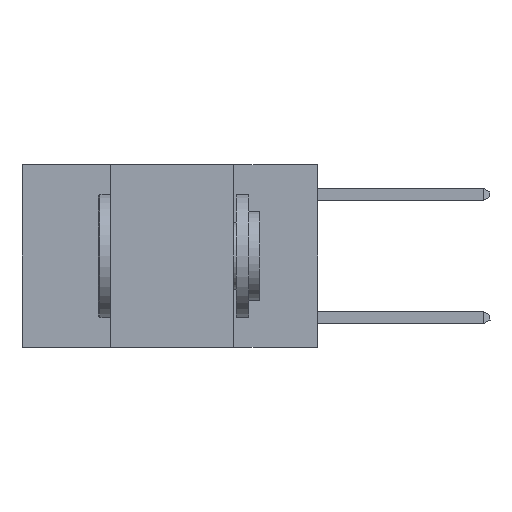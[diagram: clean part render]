
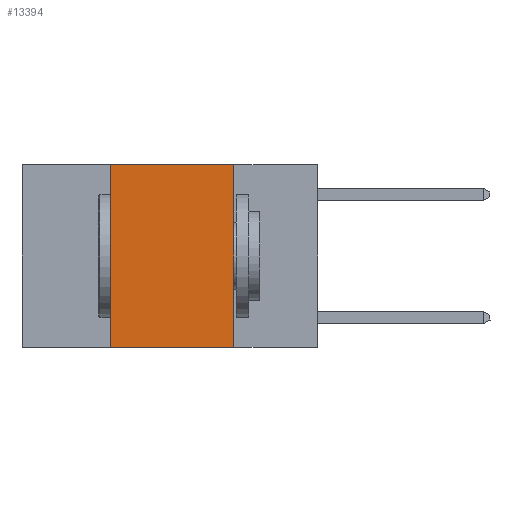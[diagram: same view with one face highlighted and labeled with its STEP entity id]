
A CAD part, left-side view. The second image highlights one B-rep face of the part: STEP entity #13394.
In plain terms, the highlighted planar face has unit normal (-1, 0, 0).
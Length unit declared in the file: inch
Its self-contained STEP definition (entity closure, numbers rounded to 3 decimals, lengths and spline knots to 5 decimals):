
#679 = LINE ( 'NONE', #3137, #19779 ) ;
#1530 = FACE_OUTER_BOUND ( 'NONE', #15177, .T. ) ;
#1655 = CARTESIAN_POINT ( 'NONE',  ( 0., 0.6, 0. ) ) ;
#1979 = CARTESIAN_POINT ( 'NONE',  ( 0., 0.6, -0.37 ) ) ;
#2832 = AXIS2_PLACEMENT_3D ( 'NONE', #16627, #18641, #7197 ) ;
#3122 = VERTEX_POINT ( 'NONE', #11796 ) ;
#3137 = CARTESIAN_POINT ( 'NONE',  ( 0., 0.42, 0. ) ) ;
#3443 = EDGE_CURVE ( 'NONE', #3122, #5852, #679, .T. ) ;
#3914 = ORIENTED_EDGE ( 'NONE', *, *, #16289, .T. ) ;
#3929 = DIRECTION ( 'NONE',  ( 0., -1., 0. ) ) ;
#4210 = VECTOR ( 'NONE', #16967, 39.37008 ) ;
#5852 = VERTEX_POINT ( 'NONE', #21834 ) ;
#7197 = DIRECTION ( 'NONE',  ( 0., 0., -1. ) ) ;
#7364 = VECTOR ( 'NONE', #3929, 39.37008 ) ;
#7994 = LINE ( 'NONE', #18593, #21418 ) ;
#8517 = CARTESIAN_POINT ( 'NONE',  ( 0., 0.17, 0. ) ) ;
#10790 = DIRECTION ( 'NONE',  ( 0., 0., 1. ) ) ;
#11796 = CARTESIAN_POINT ( 'NONE',  ( 0., 0.42, -0.37 ) ) ;
#12410 = ORIENTED_EDGE ( 'NONE', *, *, #15409, .F. ) ;
#12865 = PLANE ( 'NONE',  #2832 ) ;
#12896 = DIRECTION ( 'NONE',  ( 0., 0., -1. ) ) ;
#13394 = ADVANCED_FACE ( 'NONE', ( #1530 ), #12865, .F. ) ;
#13499 = EDGE_CURVE ( 'NONE', #5852, #18855, #13781, .T. ) ;
#13781 = LINE ( 'NONE', #1655, #4210 ) ;
#15177 = EDGE_LOOP ( 'NONE', ( #12410, #20853, #19534, #3914 ) ) ;
#15409 = EDGE_CURVE ( 'NONE', #18855, #19019, #7994, .T. ) ;
#16289 = EDGE_CURVE ( 'NONE', #3122, #19019, #22571, .T. ) ;
#16627 = CARTESIAN_POINT ( 'NONE',  ( 0., 0.6, 0. ) ) ;
#16967 = DIRECTION ( 'NONE',  ( 0., -1., 0. ) ) ;
#18593 = CARTESIAN_POINT ( 'NONE',  ( 0., 0.17, 0. ) ) ;
#18641 = DIRECTION ( 'NONE',  ( 1., 0., 0. ) ) ;
#18855 = VERTEX_POINT ( 'NONE', #8517 ) ;
#19019 = VERTEX_POINT ( 'NONE', #20531 ) ;
#19534 = ORIENTED_EDGE ( 'NONE', *, *, #3443, .F. ) ;
#19779 = VECTOR ( 'NONE', #10790, 39.37008 ) ;
#20531 = CARTESIAN_POINT ( 'NONE',  ( 0., 0.17, -0.37 ) ) ;
#20853 = ORIENTED_EDGE ( 'NONE', *, *, #13499, .F. ) ;
#21418 = VECTOR ( 'NONE', #12896, 39.37008 ) ;
#21834 = CARTESIAN_POINT ( 'NONE',  ( 0., 0.42, 0. ) ) ;
#22571 = LINE ( 'NONE', #1979, #7364 ) ;
